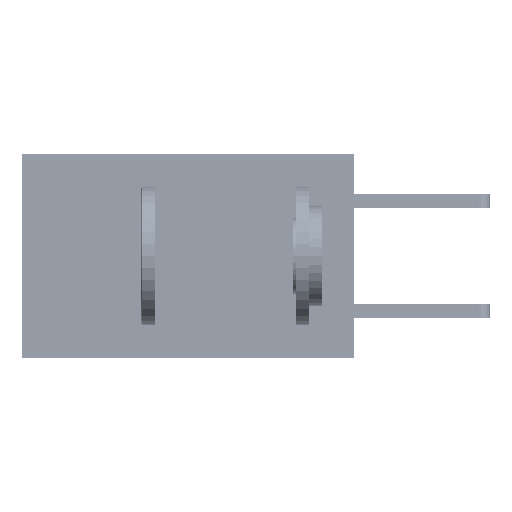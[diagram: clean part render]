
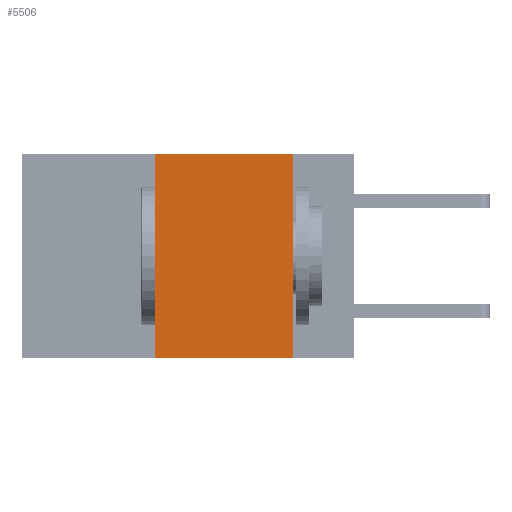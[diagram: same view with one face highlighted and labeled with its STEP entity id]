
A CAD part, left-side view. The second image highlights one B-rep face of the part: STEP entity #5506.
In plain terms, the highlighted planar face has unit normal (-1, 0, 0).
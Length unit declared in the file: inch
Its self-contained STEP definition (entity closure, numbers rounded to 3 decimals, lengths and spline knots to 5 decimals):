
#133 = EDGE_CURVE ( 'NONE', #19496, #35528, #21797, .T. ) ;
#2585 = CARTESIAN_POINT ( 'NONE',  ( 0., 0.11, 0. ) ) ;
#4401 = VECTOR ( 'NONE', #29276, 39.37008 ) ;
#5394 = ORIENTED_EDGE ( 'NONE', *, *, #34326, .F. ) ;
#5506 = ADVANCED_FACE ( 'NONE', ( #29559 ), #26175, .F. ) ;
#8460 = ORIENTED_EDGE ( 'NONE', *, *, #133, .F. ) ;
#10742 = EDGE_CURVE ( 'NONE', #28614, #35528, #11313, .T. ) ;
#11313 = LINE ( 'NONE', #25154, #40638 ) ;
#12076 = CARTESIAN_POINT ( 'NONE',  ( 0., 0.11, -0.37 ) ) ;
#14138 = VERTEX_POINT ( 'NONE', #25938 ) ;
#15363 = CARTESIAN_POINT ( 'NONE',  ( 0., 0.36, 0. ) ) ;
#15467 = DIRECTION ( 'NONE',  ( 0., -1., 0. ) ) ;
#18986 = VECTOR ( 'NONE', #15467, 39.37008 ) ;
#19496 = VERTEX_POINT ( 'NONE', #2585 ) ;
#19546 = CARTESIAN_POINT ( 'NONE',  ( 0., 0.6, 0. ) ) ;
#21797 = LINE ( 'NONE', #39699, #4401 ) ;
#22386 = LINE ( 'NONE', #15363, #27788 ) ;
#24268 = AXIS2_PLACEMENT_3D ( 'NONE', #26402, #40004, #43381 ) ;
#25154 = CARTESIAN_POINT ( 'NONE',  ( 0., 0.6, -0.37 ) ) ;
#25938 = CARTESIAN_POINT ( 'NONE',  ( 0., 0.36, 0. ) ) ;
#26175 = PLANE ( 'NONE',  #24268 ) ;
#26402 = CARTESIAN_POINT ( 'NONE',  ( 0., 0.6, 0. ) ) ;
#26658 = ORIENTED_EDGE ( 'NONE', *, *, #10742, .T. ) ;
#27788 = VECTOR ( 'NONE', #29413, 39.37008 ) ;
#28097 = CARTESIAN_POINT ( 'NONE',  ( 0., 0.36, -0.37 ) ) ;
#28614 = VERTEX_POINT ( 'NONE', #28097 ) ;
#29276 = DIRECTION ( 'NONE',  ( 0., 0., -1. ) ) ;
#29413 = DIRECTION ( 'NONE',  ( 0., 0., 1. ) ) ;
#29559 = FACE_OUTER_BOUND ( 'NONE', #43782, .T. ) ;
#34326 = EDGE_CURVE ( 'NONE', #14138, #19496, #43577, .T. ) ;
#35528 = VERTEX_POINT ( 'NONE', #12076 ) ;
#36496 = EDGE_CURVE ( 'NONE', #28614, #14138, #22386, .T. ) ;
#38534 = DIRECTION ( 'NONE',  ( 0., -1., 0. ) ) ;
#39699 = CARTESIAN_POINT ( 'NONE',  ( 0., 0.11, 0. ) ) ;
#40004 = DIRECTION ( 'NONE',  ( 1., 0., 0. ) ) ;
#40616 = ORIENTED_EDGE ( 'NONE', *, *, #36496, .F. ) ;
#40638 = VECTOR ( 'NONE', #38534, 39.37008 ) ;
#43381 = DIRECTION ( 'NONE',  ( 0., 0., -1. ) ) ;
#43577 = LINE ( 'NONE', #19546, #18986 ) ;
#43782 = EDGE_LOOP ( 'NONE', ( #8460, #5394, #40616, #26658 ) ) ;
